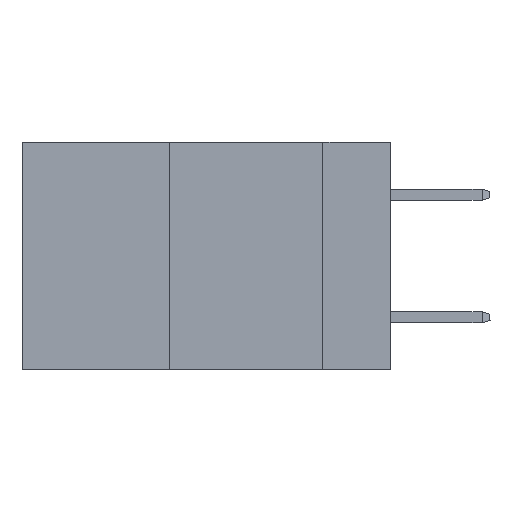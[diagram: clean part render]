
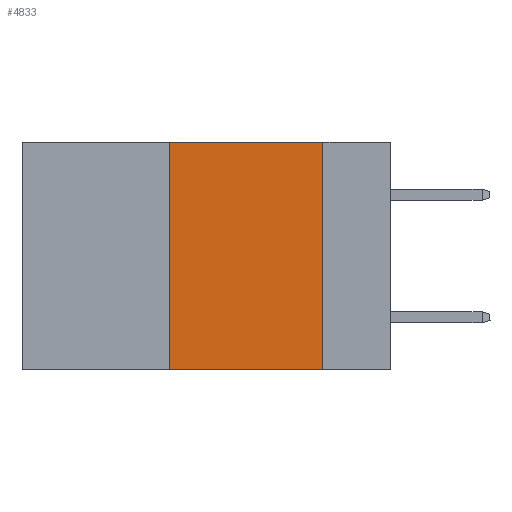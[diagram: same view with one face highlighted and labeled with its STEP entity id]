
A CAD part, left-side view. The second image highlights one B-rep face of the part: STEP entity #4833.
In plain terms, the highlighted planar face has unit normal (-1, 0, 0).
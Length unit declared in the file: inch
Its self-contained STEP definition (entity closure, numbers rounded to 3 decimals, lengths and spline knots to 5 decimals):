
#50 = CARTESIAN_POINT ( 'NONE',  ( 0., 0.11, -0.37 ) ) ;
#323 = FACE_OUTER_BOUND ( 'NONE', #21034, .T. ) ;
#458 = CARTESIAN_POINT ( 'NONE',  ( 0., 0.6, 0. ) ) ;
#1396 = DIRECTION ( 'NONE',  ( 0., 0., -1. ) ) ;
#1915 = VECTOR ( 'NONE', #5640, 39.37008 ) ;
#2487 = CARTESIAN_POINT ( 'NONE',  ( 0., 0.6, 0. ) ) ;
#3599 = EDGE_CURVE ( 'NONE', #25738, #4653, #5373, .T. ) ;
#4653 = VERTEX_POINT ( 'NONE', #50 ) ;
#4833 = ADVANCED_FACE ( 'NONE', ( #323 ), #16916, .F. ) ;
#4881 = AXIS2_PLACEMENT_3D ( 'NONE', #458, #21585, #19524 ) ;
#4987 = VECTOR ( 'NONE', #20379, 39.37008 ) ;
#5373 = LINE ( 'NONE', #11569, #27038 ) ;
#5640 = DIRECTION ( 'NONE',  ( 0., -1., 0. ) ) ;
#7136 = CARTESIAN_POINT ( 'NONE',  ( 0., 0.36, -0.37 ) ) ;
#10992 = DIRECTION ( 'NONE',  ( 0., -1., 0. ) ) ;
#11569 = CARTESIAN_POINT ( 'NONE',  ( 0., 0.11, 0. ) ) ;
#12524 = EDGE_CURVE ( 'NONE', #16037, #21414, #18727, .T. ) ;
#13589 = ORIENTED_EDGE ( 'NONE', *, *, #3599, .F. ) ;
#16037 = VERTEX_POINT ( 'NONE', #7136 ) ;
#16076 = LINE ( 'NONE', #24448, #1915 ) ;
#16537 = CARTESIAN_POINT ( 'NONE',  ( 0., 0.36, 0. ) ) ;
#16916 = PLANE ( 'NONE',  #4881 ) ;
#17298 = CARTESIAN_POINT ( 'NONE',  ( 0., 0.11, 0. ) ) ;
#17652 = ORIENTED_EDGE ( 'NONE', *, *, #25779, .F. ) ;
#18727 = LINE ( 'NONE', #16537, #4987 ) ;
#19220 = LINE ( 'NONE', #2487, #20385 ) ;
#19524 = DIRECTION ( 'NONE',  ( 0., 0., -1. ) ) ;
#20379 = DIRECTION ( 'NONE',  ( 0., 0., 1. ) ) ;
#20385 = VECTOR ( 'NONE', #10992, 39.37008 ) ;
#21034 = EDGE_LOOP ( 'NONE', ( #13589, #17652, #22435, #22247 ) ) ;
#21414 = VERTEX_POINT ( 'NONE', #23300 ) ;
#21585 = DIRECTION ( 'NONE',  ( 1., 0., 0. ) ) ;
#22247 = ORIENTED_EDGE ( 'NONE', *, *, #25562, .T. ) ;
#22435 = ORIENTED_EDGE ( 'NONE', *, *, #12524, .F. ) ;
#23300 = CARTESIAN_POINT ( 'NONE',  ( 0., 0.36, 0. ) ) ;
#24448 = CARTESIAN_POINT ( 'NONE',  ( 0., 0.6, -0.37 ) ) ;
#25562 = EDGE_CURVE ( 'NONE', #16037, #4653, #16076, .T. ) ;
#25738 = VERTEX_POINT ( 'NONE', #17298 ) ;
#25779 = EDGE_CURVE ( 'NONE', #21414, #25738, #19220, .T. ) ;
#27038 = VECTOR ( 'NONE', #1396, 39.37008 ) ;
